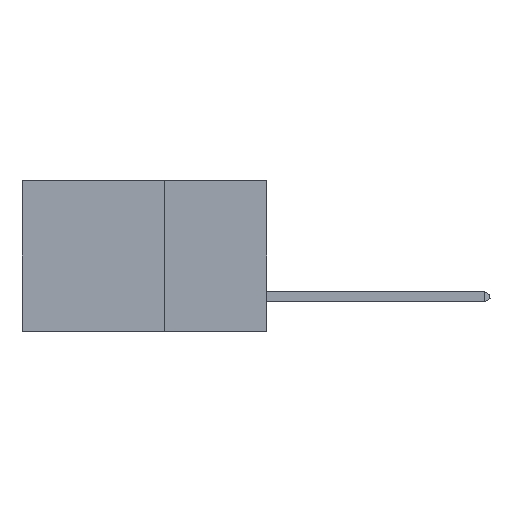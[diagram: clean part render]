
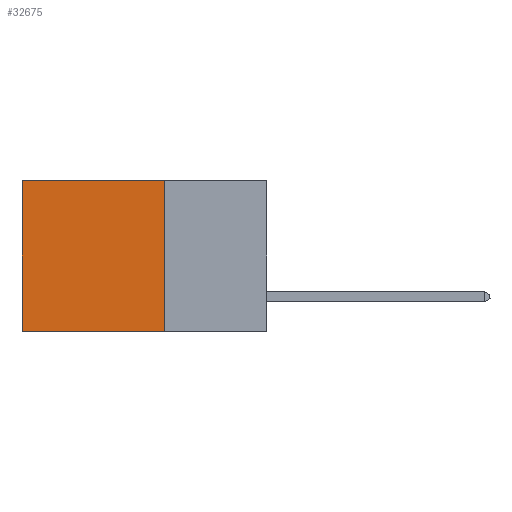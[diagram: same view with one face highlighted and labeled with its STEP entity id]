
A CAD part, left-side view. The second image highlights one B-rep face of the part: STEP entity #32675.
In plain terms, the highlighted planar face has unit normal (-1, 0, 0).
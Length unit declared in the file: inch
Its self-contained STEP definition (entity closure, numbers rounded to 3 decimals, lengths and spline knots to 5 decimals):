
#970 = CARTESIAN_POINT ( 'NONE',  ( 0.2875, 0.25, 0. ) ) ;
#1812 = VECTOR ( 'NONE', #20725, 39.37008 ) ;
#2108 = VECTOR ( 'NONE', #8953, 39.37008 ) ;
#3815 = VERTEX_POINT ( 'NONE', #16085 ) ;
#7365 = DIRECTION ( 'NONE',  ( 0., 0., -1. ) ) ;
#8953 = DIRECTION ( 'NONE',  ( 0., 1., 0. ) ) ;
#9625 = FACE_OUTER_BOUND ( 'NONE', #33785, .T. ) ;
#11287 = ORIENTED_EDGE ( 'NONE', *, *, #24328, .F. ) ;
#12350 = LINE ( 'NONE', #17812, #37582 ) ;
#13540 = DIRECTION ( 'NONE',  ( 1., 0., 0. ) ) ;
#14767 = CARTESIAN_POINT ( 'NONE',  ( 0.2875, 0.25, 0. ) ) ;
#16085 = CARTESIAN_POINT ( 'NONE',  ( 0.2875, 0.6, 0. ) ) ;
#17357 = EDGE_CURVE ( 'NONE', #28581, #3815, #12350, .T. ) ;
#17406 = ORIENTED_EDGE ( 'NONE', *, *, #17357, .T. ) ;
#17812 = CARTESIAN_POINT ( 'NONE',  ( 0.2875, 0.25, 0. ) ) ;
#17832 = VECTOR ( 'NONE', #7365, 39.37008 ) ;
#20725 = DIRECTION ( 'NONE',  ( 0., 0., -1. ) ) ;
#21025 = EDGE_CURVE ( 'NONE', #28581, #27383, #38747, .T. ) ;
#22948 = DIRECTION ( 'NONE',  ( 0., 0., -1. ) ) ;
#24328 = EDGE_CURVE ( 'NONE', #27383, #35528, #26689, .T. ) ;
#24730 = LINE ( 'NONE', #29572, #17832 ) ;
#24785 = EDGE_CURVE ( 'NONE', #3815, #35528, #24730, .T. ) ;
#26536 = PLANE ( 'NONE',  #33147 ) ;
#26689 = LINE ( 'NONE', #35842, #2108 ) ;
#27383 = VERTEX_POINT ( 'NONE', #38634 ) ;
#27868 = CARTESIAN_POINT ( 'NONE',  ( 0.2875, 0.6, -0.37 ) ) ;
#28581 = VERTEX_POINT ( 'NONE', #29006 ) ;
#29006 = CARTESIAN_POINT ( 'NONE',  ( 0.2875, 0.25, 0. ) ) ;
#29297 = ORIENTED_EDGE ( 'NONE', *, *, #24785, .T. ) ;
#29572 = CARTESIAN_POINT ( 'NONE',  ( 0.2875, 0.6, 0. ) ) ;
#32399 = DIRECTION ( 'NONE',  ( 0., 1., 0. ) ) ;
#32675 = ADVANCED_FACE ( 'NONE', ( #9625 ), #26536, .F. ) ;
#33147 = AXIS2_PLACEMENT_3D ( 'NONE', #970, #13540, #22948 ) ;
#33785 = EDGE_LOOP ( 'NONE', ( #29297, #11287, #37107, #17406 ) ) ;
#35528 = VERTEX_POINT ( 'NONE', #27868 ) ;
#35842 = CARTESIAN_POINT ( 'NONE',  ( 0.2875, 0.25, -0.37 ) ) ;
#37107 = ORIENTED_EDGE ( 'NONE', *, *, #21025, .F. ) ;
#37582 = VECTOR ( 'NONE', #32399, 39.37008 ) ;
#38634 = CARTESIAN_POINT ( 'NONE',  ( 0.2875, 0.25, -0.37 ) ) ;
#38747 = LINE ( 'NONE', #14767, #1812 ) ;
